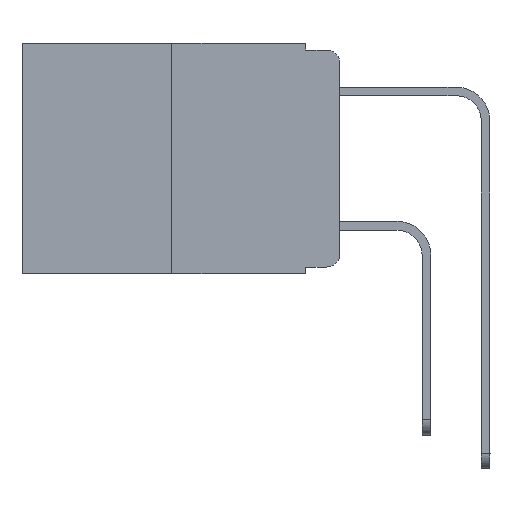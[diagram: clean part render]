
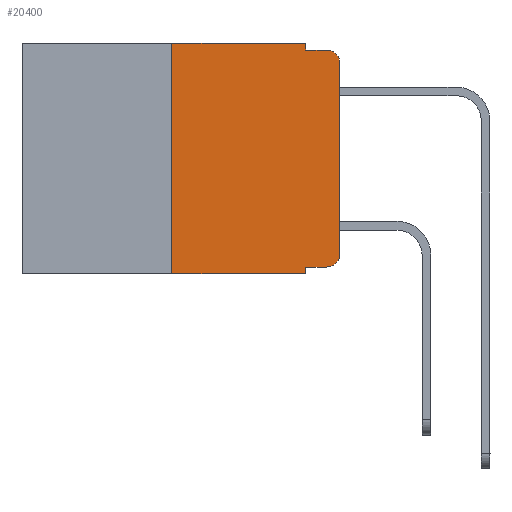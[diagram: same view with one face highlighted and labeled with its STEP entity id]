
A CAD part, left-side view. The second image highlights one B-rep face of the part: STEP entity #20400.
In plain terms, the highlighted planar face has unit normal (-1, 0, 0).
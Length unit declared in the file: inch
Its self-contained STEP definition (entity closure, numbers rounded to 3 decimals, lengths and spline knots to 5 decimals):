
#1004 = VERTEX_POINT ( 'NONE', #16371 ) ;
#1053 = LINE ( 'NONE', #9499, #11518 ) ;
#1111 = DIRECTION ( 'NONE',  ( 0., 0., -1. ) ) ;
#1221 = EDGE_CURVE ( 'NONE', #13807, #19454, #21267, .T. ) ;
#1862 = DIRECTION ( 'NONE',  ( -1., 0., 0. ) ) ;
#2170 = DIRECTION ( 'NONE',  ( 0., 0., -1. ) ) ;
#2565 = LINE ( 'NONE', #12941, #8942 ) ;
#2859 = ORIENTED_EDGE ( 'NONE', *, *, #25059, .F. ) ;
#3661 = ORIENTED_EDGE ( 'NONE', *, *, #14400, .T. ) ;
#3817 = EDGE_CURVE ( 'NONE', #19997, #24214, #11631, .T. ) ;
#3823 = VERTEX_POINT ( 'NONE', #17357 ) ;
#4321 = CIRCLE ( 'NONE', #25244, 0.02 ) ;
#4567 = ORIENTED_EDGE ( 'NONE', *, *, #8675, .T. ) ;
#5149 = VERTEX_POINT ( 'NONE', #25581 ) ;
#5263 = DIRECTION ( 'NONE',  ( -1., 0., 0. ) ) ;
#5718 = CIRCLE ( 'NONE', #9625, 0.02 ) ;
#6512 = CARTESIAN_POINT ( 'NONE',  ( 0., 0.051, -0.01 ) ) ;
#6791 = EDGE_CURVE ( 'NONE', #21347, #17905, #23232, .T. ) ;
#6808 = VECTOR ( 'NONE', #7502, 39.37008 ) ;
#6839 = CARTESIAN_POINT ( 'NONE',  ( 0., 0.473, 0. ) ) ;
#7502 = DIRECTION ( 'NONE',  ( 0., -1., 0. ) ) ;
#7548 = EDGE_CURVE ( 'NONE', #13807, #5149, #9364, .T. ) ;
#7577 = EDGE_CURVE ( 'NONE', #5149, #21347, #1053, .T. ) ;
#8235 = VECTOR ( 'NONE', #19132, 39.37008 ) ;
#8675 = EDGE_CURVE ( 'NONE', #13028, #3823, #2565, .T. ) ;
#8942 = VECTOR ( 'NONE', #14970, 39.37008 ) ;
#9302 = ORIENTED_EDGE ( 'NONE', *, *, #7548, .F. ) ;
#9364 = LINE ( 'NONE', #21923, #23264 ) ;
#9499 = CARTESIAN_POINT ( 'NONE',  ( 0., 0.473, 0. ) ) ;
#9595 = ORIENTED_EDGE ( 'NONE', *, *, #3817, .T. ) ;
#9625 = AXIS2_PLACEMENT_3D ( 'NONE', #21490, #5263, #13587 ) ;
#10307 = CARTESIAN_POINT ( 'NONE',  ( 0., 0.02, -0.313 ) ) ;
#10335 = EDGE_CURVE ( 'NONE', #13028, #19454, #16103, .T. ) ;
#10820 = CARTESIAN_POINT ( 'NONE',  ( 0., 0.051, 0. ) ) ;
#11518 = VECTOR ( 'NONE', #23429, 39.37008 ) ;
#11631 = LINE ( 'NONE', #19935, #25702 ) ;
#12093 = DIRECTION ( 'NONE',  ( 0., 0., -1. ) ) ;
#12700 = VECTOR ( 'NONE', #23710, 39.37008 ) ;
#12759 = EDGE_CURVE ( 'NONE', #3823, #19997, #4321, .T. ) ;
#12941 = CARTESIAN_POINT ( 'NONE',  ( 0., 0.051, -0.333 ) ) ;
#13028 = VERTEX_POINT ( 'NONE', #21892 ) ;
#13068 = CARTESIAN_POINT ( 'NONE',  ( 0., 0.25, -0.343 ) ) ;
#13337 = CARTESIAN_POINT ( 'NONE',  ( 0., 0., -0.03 ) ) ;
#13587 = DIRECTION ( 'NONE',  ( 0., 0., -1. ) ) ;
#13619 = DIRECTION ( 'NONE',  ( 0., 0., 1. ) ) ;
#13807 = VERTEX_POINT ( 'NONE', #13068 ) ;
#13831 = VECTOR ( 'NONE', #2170, 39.37008 ) ;
#14400 = EDGE_CURVE ( 'NONE', #24214, #1004, #5718, .T. ) ;
#14620 = AXIS2_PLACEMENT_3D ( 'NONE', #6839, #17482, #1111 ) ;
#14970 = DIRECTION ( 'NONE',  ( 0., -1., 0. ) ) ;
#15437 = PLANE ( 'NONE',  #14620 ) ;
#16103 = LINE ( 'NONE', #20855, #13831 ) ;
#16330 = ORIENTED_EDGE ( 'NONE', *, *, #10335, .F. ) ;
#16371 = CARTESIAN_POINT ( 'NONE',  ( 0., 0.02, -0.01 ) ) ;
#17357 = CARTESIAN_POINT ( 'NONE',  ( 0., 0.02, -0.333 ) ) ;
#17482 = DIRECTION ( 'NONE',  ( 1., 0., 0. ) ) ;
#17875 = CARTESIAN_POINT ( 'NONE',  ( 0., 0.051, -0.01 ) ) ;
#17905 = VERTEX_POINT ( 'NONE', #6512 ) ;
#17921 = CARTESIAN_POINT ( 'NONE',  ( 0., 0., -0.313 ) ) ;
#18446 = CARTESIAN_POINT ( 'NONE',  ( 0., 0.051, 0. ) ) ;
#18700 = ORIENTED_EDGE ( 'NONE', *, *, #1221, .T. ) ;
#19132 = DIRECTION ( 'NONE',  ( 0., 0., -1. ) ) ;
#19454 = VERTEX_POINT ( 'NONE', #23950 ) ;
#19501 = LINE ( 'NONE', #17875, #6808 ) ;
#19525 = EDGE_LOOP ( 'NONE', ( #9595, #3661, #2859, #22500, #22467, #9302, #18700, #16330, #4567, #25927 ) ) ;
#19935 = CARTESIAN_POINT ( 'NONE',  ( 0., 0., 0. ) ) ;
#19997 = VERTEX_POINT ( 'NONE', #17921 ) ;
#20400 = ADVANCED_FACE ( 'NONE', ( #23615 ), #15437, .F. ) ;
#20855 = CARTESIAN_POINT ( 'NONE',  ( 0., 0.051, 0. ) ) ;
#21267 = LINE ( 'NONE', #25760, #12700 ) ;
#21347 = VERTEX_POINT ( 'NONE', #18446 ) ;
#21490 = CARTESIAN_POINT ( 'NONE',  ( 0., 0.02, -0.03 ) ) ;
#21892 = CARTESIAN_POINT ( 'NONE',  ( 0., 0.051, -0.333 ) ) ;
#21923 = CARTESIAN_POINT ( 'NONE',  ( 0., 0.25, 0. ) ) ;
#22467 = ORIENTED_EDGE ( 'NONE', *, *, #7577, .F. ) ;
#22500 = ORIENTED_EDGE ( 'NONE', *, *, #6791, .F. ) ;
#23232 = LINE ( 'NONE', #10820, #8235 ) ;
#23264 = VECTOR ( 'NONE', #13619, 39.37008 ) ;
#23429 = DIRECTION ( 'NONE',  ( 0., -1., 0. ) ) ;
#23615 = FACE_OUTER_BOUND ( 'NONE', #19525, .T. ) ;
#23710 = DIRECTION ( 'NONE',  ( 0., -1., 0. ) ) ;
#23767 = DIRECTION ( 'NONE',  ( 0., 0., 1. ) ) ;
#23950 = CARTESIAN_POINT ( 'NONE',  ( 0., 0.051, -0.343 ) ) ;
#24214 = VERTEX_POINT ( 'NONE', #13337 ) ;
#25059 = EDGE_CURVE ( 'NONE', #17905, #1004, #19501, .T. ) ;
#25244 = AXIS2_PLACEMENT_3D ( 'NONE', #10307, #1862, #12093 ) ;
#25581 = CARTESIAN_POINT ( 'NONE',  ( 0., 0.25, 0. ) ) ;
#25702 = VECTOR ( 'NONE', #23767, 39.37008 ) ;
#25760 = CARTESIAN_POINT ( 'NONE',  ( 0., 0.473, -0.343 ) ) ;
#25927 = ORIENTED_EDGE ( 'NONE', *, *, #12759, .T. ) ;
